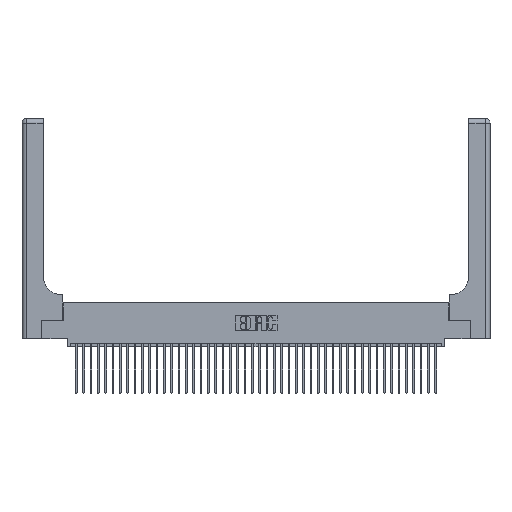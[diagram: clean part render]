
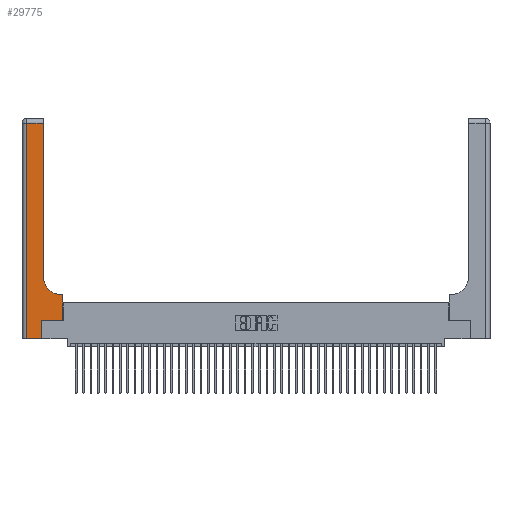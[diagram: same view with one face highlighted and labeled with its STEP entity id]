
A CAD part, top view. The second image highlights one B-rep face of the part: STEP entity #29775.
In plain terms, the highlighted planar face has unit normal (0, 0, 1).
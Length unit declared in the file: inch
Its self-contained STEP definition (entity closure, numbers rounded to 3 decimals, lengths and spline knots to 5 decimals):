
#728 = DIRECTION ( 'NONE',  ( -1., 0., 0. ) ) ;
#763 = LINE ( 'NONE', #29970, #16637 ) ;
#1151 = CARTESIAN_POINT ( 'NONE',  ( 0.2915, 3., 0.37 ) ) ;
#1238 = DIRECTION ( 'NONE',  ( -1., 0., 0. ) ) ;
#2420 = LINE ( 'NONE', #20937, #38163 ) ;
#2640 = AXIS2_PLACEMENT_3D ( 'NONE', #18089, #21449, #1238 ) ;
#2759 = CARTESIAN_POINT ( 'NONE',  ( 0.269, 0., 0.37 ) ) ;
#2811 = VERTEX_POINT ( 'NONE', #6866 ) ;
#3586 = FACE_OUTER_BOUND ( 'NONE', #40484, .T. ) ;
#3795 = VERTEX_POINT ( 'NONE', #22572 ) ;
#4060 = LINE ( 'NONE', #23783, #29877 ) ;
#5592 = CARTESIAN_POINT ( 'NONE',  ( 0.269, 0., 0.37 ) ) ;
#5633 = ORIENTED_EDGE ( 'NONE', *, *, #19237, .T. ) ;
#6664 = EDGE_CURVE ( 'NONE', #2811, #23721, #32964, .T. ) ;
#6866 = CARTESIAN_POINT ( 'NONE',  ( 0.269, 0.25, 0.37 ) ) ;
#7696 = CARTESIAN_POINT ( 'NONE',  ( 0.5585, 0.25, 0.37 ) ) ;
#9046 = CARTESIAN_POINT ( 'NONE',  ( 0.5585, 0.25, 0.37 ) ) ;
#9833 = VERTEX_POINT ( 'NONE', #18123 ) ;
#10546 = VERTEX_POINT ( 'NONE', #31673 ) ;
#10552 = ORIENTED_EDGE ( 'NONE', *, *, #6664, .T. ) ;
#11167 = CARTESIAN_POINT ( 'NONE',  ( 0.06, 2.94, 0.37 ) ) ;
#14231 = ORIENTED_EDGE ( 'NONE', *, *, #18417, .T. ) ;
#15004 = CARTESIAN_POINT ( 'NONE',  ( 0., 0., 0.37 ) ) ;
#15680 = CARTESIAN_POINT ( 'NONE',  ( 0.5415, 0.6, 0.37 ) ) ;
#15723 = LINE ( 'NONE', #1151, #32490 ) ;
#15913 = CARTESIAN_POINT ( 'NONE',  ( 0.2915, 0.85, 0.37 ) ) ;
#15952 = EDGE_CURVE ( 'NONE', #28661, #40652, #32715, .T. ) ;
#16637 = VECTOR ( 'NONE', #40044, 39.37008 ) ;
#17426 = VERTEX_POINT ( 'NONE', #11167 ) ;
#18089 = CARTESIAN_POINT ( 'NONE',  ( 0., 3., 0.37 ) ) ;
#18123 = CARTESIAN_POINT ( 'NONE',  ( 0.2915, 2.94, 0.37 ) ) ;
#18417 = EDGE_CURVE ( 'NONE', #23721, #3795, #25167, .T. ) ;
#18477 = EDGE_CURVE ( 'NONE', #17426, #10546, #4060, .T. ) ;
#18604 = AXIS2_PLACEMENT_3D ( 'NONE', #19929, #43340, #23323 ) ;
#18610 = ORIENTED_EDGE ( 'NONE', *, *, #15952, .T. ) ;
#19237 = EDGE_CURVE ( 'NONE', #9833, #17426, #2420, .T. ) ;
#19590 = VERTEX_POINT ( 'NONE', #2759 ) ;
#19929 = CARTESIAN_POINT ( 'NONE',  ( 0.5415, 0.85, 0.37 ) ) ;
#20937 = CARTESIAN_POINT ( 'NONE',  ( 0., 2.94, 0.37 ) ) ;
#21449 = DIRECTION ( 'NONE',  ( 0., 0., -1. ) ) ;
#22572 = CARTESIAN_POINT ( 'NONE',  ( 0.5585, 0.6, 0.37 ) ) ;
#23323 = DIRECTION ( 'NONE',  ( 1., 0., 0. ) ) ;
#23721 = VERTEX_POINT ( 'NONE', #7696 ) ;
#23783 = CARTESIAN_POINT ( 'NONE',  ( 0.06, 3., 0.37 ) ) ;
#24068 = VECTOR ( 'NONE', #27758, 39.37008 ) ;
#24256 = ORIENTED_EDGE ( 'NONE', *, *, #31899, .T. ) ;
#24420 = CARTESIAN_POINT ( 'NONE',  ( 0.269, 0.25, 0.37 ) ) ;
#25146 = VECTOR ( 'NONE', #29103, 39.37008 ) ;
#25167 = LINE ( 'NONE', #9046, #41910 ) ;
#27121 = DIRECTION ( 'NONE',  ( 0., -1., 0. ) ) ;
#27577 = ORIENTED_EDGE ( 'NONE', *, *, #37920, .T. ) ;
#27758 = DIRECTION ( 'NONE',  ( 1., 0., 0. ) ) ;
#28661 = VERTEX_POINT ( 'NONE', #15680 ) ;
#29103 = DIRECTION ( 'NONE',  ( 0., 1., 0. ) ) ;
#29775 = ADVANCED_FACE ( 'NONE', ( #3586 ), #38115, .F. ) ;
#29877 = VECTOR ( 'NONE', #27121, 39.37008 ) ;
#29970 = CARTESIAN_POINT ( 'NONE',  ( 0.2915, 0.6, 0.37 ) ) ;
#30170 = LINE ( 'NONE', #15004, #37990 ) ;
#30842 = ORIENTED_EDGE ( 'NONE', *, *, #37708, .T. ) ;
#31160 = ORIENTED_EDGE ( 'NONE', *, *, #18477, .T. ) ;
#31673 = CARTESIAN_POINT ( 'NONE',  ( 0.06, 0., 0.37 ) ) ;
#31695 = DIRECTION ( 'NONE',  ( 1., 0., 0. ) ) ;
#31899 = EDGE_CURVE ( 'NONE', #3795, #28661, #763, .T. ) ;
#32490 = VECTOR ( 'NONE', #38180, 39.37008 ) ;
#32715 = CIRCLE ( 'NONE', #18604, 0.25 ) ;
#32964 = LINE ( 'NONE', #24420, #24068 ) ;
#33753 = EDGE_CURVE ( 'NONE', #10546, #19590, #30170, .T. ) ;
#37708 = EDGE_CURVE ( 'NONE', #40652, #9833, #15723, .T. ) ;
#37920 = EDGE_CURVE ( 'NONE', #19590, #2811, #42956, .T. ) ;
#37990 = VECTOR ( 'NONE', #31695, 39.37008 ) ;
#38115 = PLANE ( 'NONE',  #2640 ) ;
#38163 = VECTOR ( 'NONE', #728, 39.37008 ) ;
#38180 = DIRECTION ( 'NONE',  ( 0., 1., 0. ) ) ;
#39204 = DIRECTION ( 'NONE',  ( 0., 1., 0. ) ) ;
#40044 = DIRECTION ( 'NONE',  ( -1., 0., 0. ) ) ;
#40484 = EDGE_LOOP ( 'NONE', ( #30842, #5633, #31160, #43259, #27577, #10552, #14231, #24256, #18610 ) ) ;
#40652 = VERTEX_POINT ( 'NONE', #15913 ) ;
#41910 = VECTOR ( 'NONE', #39204, 39.37008 ) ;
#42956 = LINE ( 'NONE', #5592, #25146 ) ;
#43259 = ORIENTED_EDGE ( 'NONE', *, *, #33753, .T. ) ;
#43340 = DIRECTION ( 'NONE',  ( 0., 0., -1. ) ) ;
